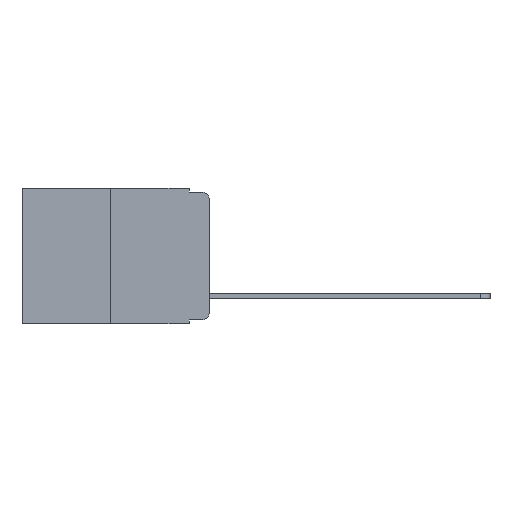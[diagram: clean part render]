
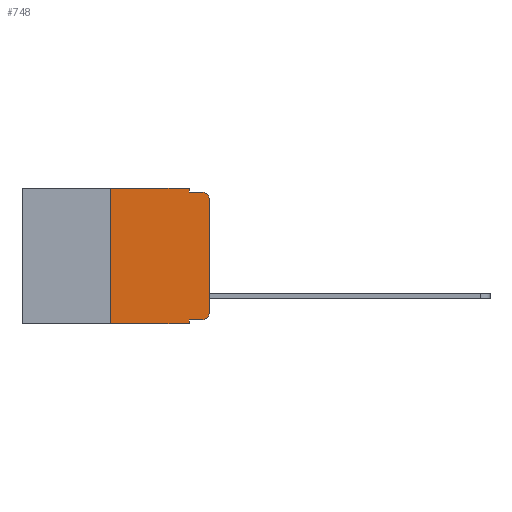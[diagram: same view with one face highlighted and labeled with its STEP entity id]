
A CAD part, left-side view. The second image highlights one B-rep face of the part: STEP entity #748.
In plain terms, the highlighted planar face has unit normal (-1, 0, 0).
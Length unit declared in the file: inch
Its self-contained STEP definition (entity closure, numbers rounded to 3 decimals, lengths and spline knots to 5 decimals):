
#290 = LINE ( 'NONE', #14004, #7768 ) ;
#488 = VECTOR ( 'NONE', #10941, 39.37008 ) ;
#499 = LINE ( 'NONE', #10701, #14487 ) ;
#748 = ADVANCED_FACE ( 'NONE', ( #14175 ), #15174, .F. ) ;
#1101 = DIRECTION ( 'NONE',  ( 0., 0., 1. ) ) ;
#1123 = ORIENTED_EDGE ( 'NONE', *, *, #12847, .F. ) ;
#1703 = EDGE_CURVE ( 'NONE', #4044, #5006, #5222, .T. ) ;
#1912 = DIRECTION ( 'NONE',  ( -1., 0., 0. ) ) ;
#1931 = CARTESIAN_POINT ( 'NONE',  ( 0., 0.02, -0.313 ) ) ;
#2304 = EDGE_CURVE ( 'NONE', #3569, #4297, #8646, .T. ) ;
#2737 = CARTESIAN_POINT ( 'NONE',  ( 0., 0., -0.313 ) ) ;
#2851 = CARTESIAN_POINT ( 'NONE',  ( 0., 0.051, -0.01 ) ) ;
#2921 = ORIENTED_EDGE ( 'NONE', *, *, #1703, .T. ) ;
#3037 = LINE ( 'NONE', #2851, #8642 ) ;
#3104 = LINE ( 'NONE', #15028, #16802 ) ;
#3495 = CARTESIAN_POINT ( 'NONE',  ( 0., 0.02, -0.333 ) ) ;
#3569 = VERTEX_POINT ( 'NONE', #14001 ) ;
#4044 = VERTEX_POINT ( 'NONE', #3495 ) ;
#4165 = CARTESIAN_POINT ( 'NONE',  ( 0., 0.051, -0.333 ) ) ;
#4201 = VERTEX_POINT ( 'NONE', #6535 ) ;
#4245 = VECTOR ( 'NONE', #15695, 39.37008 ) ;
#4297 = VERTEX_POINT ( 'NONE', #11966 ) ;
#4481 = CARTESIAN_POINT ( 'NONE',  ( 0., 0.051, -0.333 ) ) ;
#4830 = VECTOR ( 'NONE', #11248, 39.37008 ) ;
#5006 = VERTEX_POINT ( 'NONE', #2737 ) ;
#5222 = CIRCLE ( 'NONE', #11764, 0.02 ) ;
#5335 = VERTEX_POINT ( 'NONE', #6844 ) ;
#5412 = VERTEX_POINT ( 'NONE', #4165 ) ;
#5545 = EDGE_CURVE ( 'NONE', #10512, #16797, #3104, .T. ) ;
#6208 = DIRECTION ( 'NONE',  ( 0., 0., -1. ) ) ;
#6535 = CARTESIAN_POINT ( 'NONE',  ( 0., 0.051, -0.01 ) ) ;
#6629 = ORIENTED_EDGE ( 'NONE', *, *, #11953, .F. ) ;
#6844 = CARTESIAN_POINT ( 'NONE',  ( 0., 0.25, -0.343 ) ) ;
#7316 = VECTOR ( 'NONE', #12008, 39.37008 ) ;
#7498 = DIRECTION ( 'NONE',  ( 0., 0., -1. ) ) ;
#7768 = VECTOR ( 'NONE', #7498, 39.37008 ) ;
#7919 = ORIENTED_EDGE ( 'NONE', *, *, #5545, .F. ) ;
#7943 = LINE ( 'NONE', #9656, #488 ) ;
#8489 = LINE ( 'NONE', #4481, #4830 ) ;
#8642 = VECTOR ( 'NONE', #12301, 39.37008 ) ;
#8646 = CIRCLE ( 'NONE', #11988, 0.02 ) ;
#9264 = CARTESIAN_POINT ( 'NONE',  ( 0., 0.051, 0. ) ) ;
#9656 = CARTESIAN_POINT ( 'NONE',  ( 0., 0.473, -0.343 ) ) ;
#9705 = DIRECTION ( 'NONE',  ( 0., 0., -1. ) ) ;
#9890 = DIRECTION ( 'NONE',  ( 0., -1., 0. ) ) ;
#10008 = EDGE_CURVE ( 'NONE', #5335, #10512, #10418, .T. ) ;
#10418 = LINE ( 'NONE', #10698, #7316 ) ;
#10512 = VERTEX_POINT ( 'NONE', #16944 ) ;
#10531 = EDGE_CURVE ( 'NONE', #16797, #4201, #14847, .T. ) ;
#10698 = CARTESIAN_POINT ( 'NONE',  ( 0., 0.25, 0. ) ) ;
#10701 = CARTESIAN_POINT ( 'NONE',  ( 0., 0., 0. ) ) ;
#10941 = DIRECTION ( 'NONE',  ( 0., -1., 0. ) ) ;
#11248 = DIRECTION ( 'NONE',  ( 0., -1., 0. ) ) ;
#11409 = ORIENTED_EDGE ( 'NONE', *, *, #10008, .F. ) ;
#11764 = AXIS2_PLACEMENT_3D ( 'NONE', #1931, #1912, #17229 ) ;
#11953 = EDGE_CURVE ( 'NONE', #4201, #4297, #3037, .T. ) ;
#11966 = CARTESIAN_POINT ( 'NONE',  ( 0., 0.02, -0.01 ) ) ;
#11988 = AXIS2_PLACEMENT_3D ( 'NONE', #15299, #17334, #6208 ) ;
#11998 = ORIENTED_EDGE ( 'NONE', *, *, #15384, .T. ) ;
#12008 = DIRECTION ( 'NONE',  ( 0., 0., 1. ) ) ;
#12020 = ORIENTED_EDGE ( 'NONE', *, *, #16606, .T. ) ;
#12301 = DIRECTION ( 'NONE',  ( 0., -1., 0. ) ) ;
#12706 = CARTESIAN_POINT ( 'NONE',  ( 0., 0.051, -0.343 ) ) ;
#12845 = ORIENTED_EDGE ( 'NONE', *, *, #2304, .T. ) ;
#12847 = EDGE_CURVE ( 'NONE', #5412, #13413, #290, .T. ) ;
#13173 = EDGE_CURVE ( 'NONE', #5335, #13413, #7943, .T. ) ;
#13413 = VERTEX_POINT ( 'NONE', #12706 ) ;
#13718 = DIRECTION ( 'NONE',  ( 1., 0., 0. ) ) ;
#14001 = CARTESIAN_POINT ( 'NONE',  ( 0., 0., -0.03 ) ) ;
#14004 = CARTESIAN_POINT ( 'NONE',  ( 0., 0.051, 0. ) ) ;
#14036 = ORIENTED_EDGE ( 'NONE', *, *, #10531, .F. ) ;
#14175 = FACE_OUTER_BOUND ( 'NONE', #16162, .T. ) ;
#14223 = CARTESIAN_POINT ( 'NONE',  ( 0., 0.473, 0. ) ) ;
#14487 = VECTOR ( 'NONE', #1101, 39.37008 ) ;
#14847 = LINE ( 'NONE', #9264, #4245 ) ;
#15025 = ORIENTED_EDGE ( 'NONE', *, *, #13173, .T. ) ;
#15028 = CARTESIAN_POINT ( 'NONE',  ( 0., 0.473, 0. ) ) ;
#15174 = PLANE ( 'NONE',  #15324 ) ;
#15299 = CARTESIAN_POINT ( 'NONE',  ( 0., 0.02, -0.03 ) ) ;
#15324 = AXIS2_PLACEMENT_3D ( 'NONE', #14223, #13718, #9705 ) ;
#15384 = EDGE_CURVE ( 'NONE', #5412, #4044, #8489, .T. ) ;
#15695 = DIRECTION ( 'NONE',  ( 0., 0., -1. ) ) ;
#16162 = EDGE_LOOP ( 'NONE', ( #12020, #12845, #6629, #14036, #7919, #11409, #15025, #1123, #11998, #2921 ) ) ;
#16281 = CARTESIAN_POINT ( 'NONE',  ( 0., 0.051, 0. ) ) ;
#16606 = EDGE_CURVE ( 'NONE', #5006, #3569, #499, .T. ) ;
#16797 = VERTEX_POINT ( 'NONE', #16281 ) ;
#16802 = VECTOR ( 'NONE', #9890, 39.37008 ) ;
#16944 = CARTESIAN_POINT ( 'NONE',  ( 0., 0.25, 0. ) ) ;
#17229 = DIRECTION ( 'NONE',  ( 0., 0., -1. ) ) ;
#17334 = DIRECTION ( 'NONE',  ( -1., 0., 0. ) ) ;
